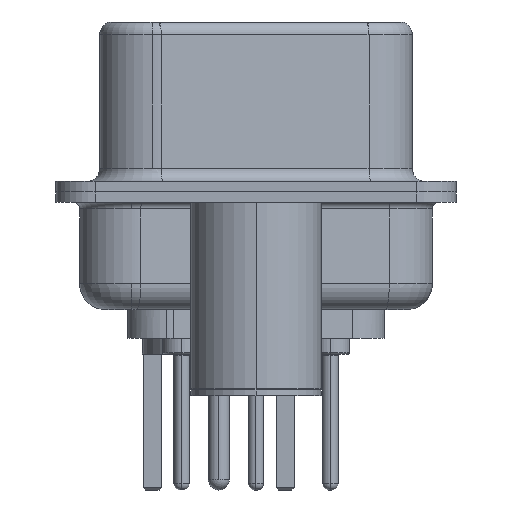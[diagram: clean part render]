
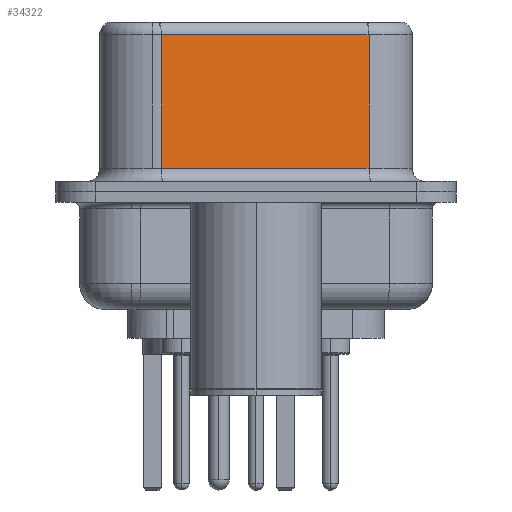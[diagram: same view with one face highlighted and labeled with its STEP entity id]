
A CAD part, left-side view. The second image highlights one B-rep face of the part: STEP entity #34322.
In plain terms, the highlighted planar face has unit normal (-0.985, -0.174, 0).
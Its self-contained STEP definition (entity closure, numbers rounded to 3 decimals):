
#285 = CARTESIAN_POINT ( 'NONE',  ( 5.132, -4.322, 0.9 ) ) ;
#1274 = ORIENTED_EDGE ( 'NONE', *, *, #34349, .T. ) ;
#2029 = DIRECTION ( 'NONE',  ( 0.985, 0.174, 0. ) ) ;
#2213 = CARTESIAN_POINT ( 'NONE',  ( 3.73, 3.628, 6.02 ) ) ;
#2921 = LINE ( 'NONE', #9456, #29675 ) ;
#3591 = CARTESIAN_POINT ( 'NONE',  ( 3.73, 3.628, 0.9 ) ) ;
#4319 = DIRECTION ( 'NONE',  ( 0.174, -0.985, 0. ) ) ;
#5774 = LINE ( 'NONE', #16289, #32090 ) ;
#6245 = VERTEX_POINT ( 'NONE', #285 ) ;
#6704 = EDGE_LOOP ( 'NONE', ( #15590, #1274, #26769, #22592 ) ) ;
#7059 = CARTESIAN_POINT ( 'NONE',  ( 3.73, 3.628, 6.52 ) ) ;
#7302 = PLANE ( 'NONE',  #32422 ) ;
#7729 = FACE_OUTER_BOUND ( 'NONE', #6704, .T. ) ;
#9456 = CARTESIAN_POINT ( 'NONE',  ( 5.132, -4.322, 0.9 ) ) ;
#11198 = LINE ( 'NONE', #7059, #16472 ) ;
#12565 = LINE ( 'NONE', #12935, #27028 ) ;
#12935 = CARTESIAN_POINT ( 'NONE',  ( 5.132, -4.322, 6.02 ) ) ;
#13158 = VERTEX_POINT ( 'NONE', #2213 ) ;
#14539 = EDGE_CURVE ( 'NONE', #13158, #34841, #11198, .T. ) ;
#15009 = EDGE_CURVE ( 'NONE', #34841, #6245, #2921, .T. ) ;
#15590 = ORIENTED_EDGE ( 'NONE', *, *, #23161, .F. ) ;
#15869 = CARTESIAN_POINT ( 'NONE',  ( 5.132, -4.322, 6.52 ) ) ;
#16289 = CARTESIAN_POINT ( 'NONE',  ( 5.132, -4.322, 6.52 ) ) ;
#16472 = VECTOR ( 'NONE', #26656, 1000. ) ;
#16540 = DIRECTION ( 'NONE',  ( 0., 0., -1. ) ) ;
#22592 = ORIENTED_EDGE ( 'NONE', *, *, #15009, .T. ) ;
#23161 = EDGE_CURVE ( 'NONE', #29974, #6245, #5774, .T. ) ;
#23920 = DIRECTION ( 'NONE',  ( -0.174, 0.985, 0. ) ) ;
#24160 = DIRECTION ( 'NONE',  ( -0.174, 0.985, 0. ) ) ;
#26656 = DIRECTION ( 'NONE',  ( 0., 0., -1. ) ) ;
#26769 = ORIENTED_EDGE ( 'NONE', *, *, #14539, .T. ) ;
#27028 = VECTOR ( 'NONE', #23920, 1000. ) ;
#27584 = CARTESIAN_POINT ( 'NONE',  ( 5.132, -4.322, 6.02 ) ) ;
#29675 = VECTOR ( 'NONE', #4319, 1000. ) ;
#29974 = VERTEX_POINT ( 'NONE', #27584 ) ;
#32090 = VECTOR ( 'NONE', #16540, 1000. ) ;
#32422 = AXIS2_PLACEMENT_3D ( 'NONE', #15869, #2029, #24160 ) ;
#34322 = ADVANCED_FACE ( 'NONE', ( #7729 ), #7302, .F. ) ;
#34349 = EDGE_CURVE ( 'NONE', #29974, #13158, #12565, .T. ) ;
#34841 = VERTEX_POINT ( 'NONE', #3591 ) ;
